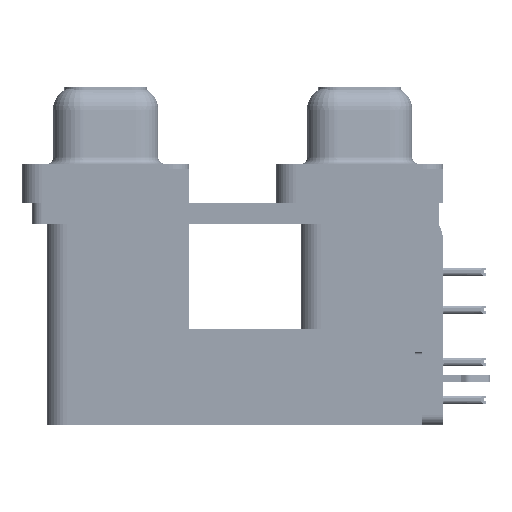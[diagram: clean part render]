
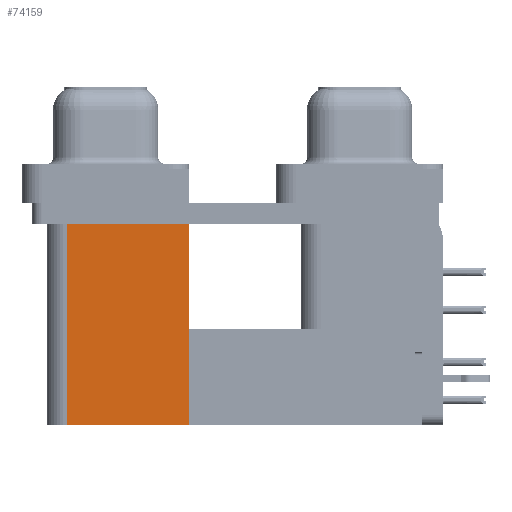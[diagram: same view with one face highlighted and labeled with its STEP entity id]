
A CAD part, left-side view. The second image highlights one B-rep face of the part: STEP entity #74159.
In plain terms, the highlighted planar face has unit normal (-1, 0, 0).
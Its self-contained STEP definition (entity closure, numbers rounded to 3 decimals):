
#1579 = VECTOR ( 'NONE', #38855, 1000. ) ;
#1839 = CARTESIAN_POINT ( 'NONE',  ( 3.79, 12.775, -19.2 ) ) ;
#5312 = EDGE_CURVE ( 'NONE', #20165, #46647, #57988, .T. ) ;
#7869 = EDGE_CURVE ( 'NONE', #17485, #56290, #23700, .T. ) ;
#9170 = CARTESIAN_POINT ( 'NONE',  ( 3.79, 12.775, -2.5 ) ) ;
#10050 = CARTESIAN_POINT ( 'NONE',  ( 3.79, 21.975, -19.2 ) ) ;
#11731 = AXIS2_PLACEMENT_3D ( 'NONE', #35152, #24361, #29362 ) ;
#13225 = DIRECTION ( 'NONE',  ( 0., 1., 0. ) ) ;
#17458 = PLANE ( 'NONE',  #11731 ) ;
#17485 = VERTEX_POINT ( 'NONE', #1839 ) ;
#17678 = LINE ( 'NONE', #24204, #41870 ) ;
#19591 = VECTOR ( 'NONE', #13225, 1000. ) ;
#20165 = VERTEX_POINT ( 'NONE', #9170 ) ;
#21526 = LINE ( 'NONE', #38087, #1579 ) ;
#23700 = LINE ( 'NONE', #64961, #66707 ) ;
#23822 = DIRECTION ( 'NONE',  ( 0., 0., 1. ) ) ;
#24204 = CARTESIAN_POINT ( 'NONE',  ( 3.79, 21.975, -19.2 ) ) ;
#24361 = DIRECTION ( 'NONE',  ( 1., 0., 0. ) ) ;
#26157 = ORIENTED_EDGE ( 'NONE', *, *, #5312, .T. ) ;
#27740 = CARTESIAN_POINT ( 'NONE',  ( 3.79, 21.975, -2.5 ) ) ;
#29362 = DIRECTION ( 'NONE',  ( 0., 0., -1. ) ) ;
#31678 = ORIENTED_EDGE ( 'NONE', *, *, #52530, .T. ) ;
#35152 = CARTESIAN_POINT ( 'NONE',  ( 3.79, 12.775, -19.2 ) ) ;
#35834 = ORIENTED_EDGE ( 'NONE', *, *, #37575, .F. ) ;
#37575 = EDGE_CURVE ( 'NONE', #56290, #46647, #17678, .T. ) ;
#38087 = CARTESIAN_POINT ( 'NONE',  ( 3.79, 12.775, -19.2 ) ) ;
#38855 = DIRECTION ( 'NONE',  ( 0., 0., 1. ) ) ;
#40641 = DIRECTION ( 'NONE',  ( 0., 1., 0. ) ) ;
#41870 = VECTOR ( 'NONE', #23822, 1000. ) ;
#46647 = VERTEX_POINT ( 'NONE', #27740 ) ;
#46741 = FACE_OUTER_BOUND ( 'NONE', #54913, .T. ) ;
#48287 = ORIENTED_EDGE ( 'NONE', *, *, #7869, .F. ) ;
#52530 = EDGE_CURVE ( 'NONE', #17485, #20165, #21526, .T. ) ;
#54913 = EDGE_LOOP ( 'NONE', ( #26157, #35834, #48287, #31678 ) ) ;
#56290 = VERTEX_POINT ( 'NONE', #10050 ) ;
#57988 = LINE ( 'NONE', #69980, #19591 ) ;
#64961 = CARTESIAN_POINT ( 'NONE',  ( 3.79, 12.775, -19.2 ) ) ;
#66707 = VECTOR ( 'NONE', #40641, 1000. ) ;
#69980 = CARTESIAN_POINT ( 'NONE',  ( 3.79, 12.775, -2.5 ) ) ;
#74159 = ADVANCED_FACE ( 'NONE', ( #46741 ), #17458, .F. ) ;
